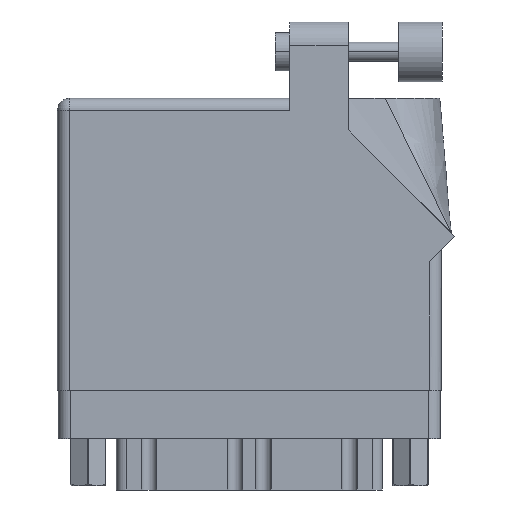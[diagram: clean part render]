
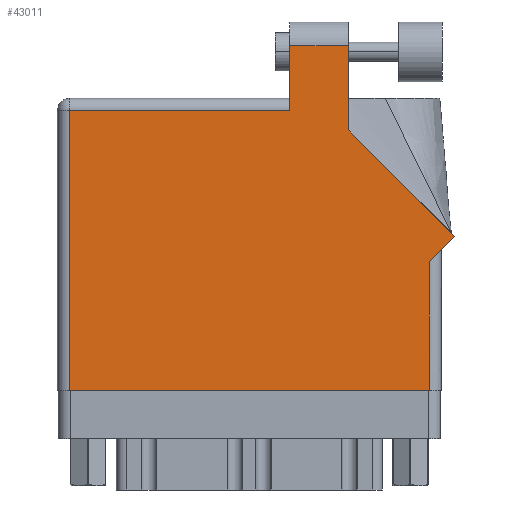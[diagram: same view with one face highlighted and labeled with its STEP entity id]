
A CAD part, front view. The second image highlights one B-rep face of the part: STEP entity #43011.
In plain terms, the highlighted face is planar.
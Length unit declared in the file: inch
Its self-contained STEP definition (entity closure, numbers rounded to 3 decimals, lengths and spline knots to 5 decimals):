
#286 = LINE ( 'NONE', #14933, #8045 ) ;
#1518 = VERTEX_POINT ( 'NONE', #29325 ) ;
#2698 = LINE ( 'NONE', #29049, #46288 ) ;
#2774 = CARTESIAN_POINT ( 'NONE',  ( 1.948, 0.737, 0. ) ) ;
#3242 = VERTEX_POINT ( 'NONE', #34035 ) ;
#4412 = LINE ( 'NONE', #15689, #27110 ) ;
#5525 = CARTESIAN_POINT ( 'NONE',  ( 1.524, 1.36442, 0. ) ) ;
#5708 = CARTESIAN_POINT ( 'NONE',  ( 1.948, 0.675, 0. ) ) ;
#6095 = EDGE_CURVE ( 'NONE', #1518, #3242, #2698, .T. ) ;
#6909 = DIRECTION ( 'NONE',  ( -1., 0., 0. ) ) ;
#7051 = CARTESIAN_POINT ( 'NONE',  ( 2.08071, 0.80771, 0. ) ) ;
#7114 = CARTESIAN_POINT ( 'NONE',  ( 0.062, 0., 0. ) ) ;
#7237 = DIRECTION ( 'NONE',  ( 0., -1., 0. ) ) ;
#7790 = EDGE_CURVE ( 'NONE', #12646, #35884, #40421, .T. ) ;
#7879 = EDGE_CURVE ( 'NONE', #41686, #40279, #4412, .T. ) ;
#8045 = VECTOR ( 'NONE', #7237, 39.37008 ) ;
#8227 = DIRECTION ( 'NONE',  ( -1., 0., 0. ) ) ;
#8655 = EDGE_CURVE ( 'NONE', #35884, #24868, #16354, .T. ) ;
#9692 = CARTESIAN_POINT ( 'NONE',  ( 0., 1.53, 0. ) ) ;
#9715 = ORIENTED_EDGE ( 'NONE', *, *, #6095, .T. ) ;
#9920 = ORIENTED_EDGE ( 'NONE', *, *, #22254, .T. ) ;
#10200 = LINE ( 'NONE', #2774, #47180 ) ;
#11770 = VECTOR ( 'NONE', #32946, 39.37008 ) ;
#12646 = VERTEX_POINT ( 'NONE', #17218 ) ;
#13825 = ORIENTED_EDGE ( 'NONE', *, *, #7879, .T. ) ;
#14439 = DIRECTION ( 'NONE',  ( 1., 0., 0. ) ) ;
#14933 = CARTESIAN_POINT ( 'NONE',  ( 1.217, 1.53, 0. ) ) ;
#15599 = VECTOR ( 'NONE', #21138, 39.37008 ) ;
#15689 = CARTESIAN_POINT ( 'NONE',  ( 0., 1.468, 0. ) ) ;
#16354 = LINE ( 'NONE', #5525, #38835 ) ;
#17140 = PLANE ( 'NONE',  #17271 ) ;
#17218 = CARTESIAN_POINT ( 'NONE',  ( 2.08071, 0.80771, 0. ) ) ;
#17271 = AXIS2_PLACEMENT_3D ( 'NONE', #9692, #24338, #28176 ) ;
#18634 = EDGE_LOOP ( 'NONE', ( #26351, #27932, #33736, #13825, #19053, #9715, #9920, #35717, #26073 ) ) ;
#19053 = ORIENTED_EDGE ( 'NONE', *, *, #24812, .T. ) ;
#19126 = CARTESIAN_POINT ( 'NONE',  ( 0.062, 1.468, 0. ) ) ;
#19299 = EDGE_CURVE ( 'NONE', #30271, #12646, #25188, .T. ) ;
#21138 = DIRECTION ( 'NONE',  ( 0.707, 0.707, 0. ) ) ;
#22254 = EDGE_CURVE ( 'NONE', #3242, #30271, #10200, .T. ) ;
#22454 = VECTOR ( 'NONE', #6909, 39.37008 ) ;
#24338 = DIRECTION ( 'NONE',  ( 0., 0., -1. ) ) ;
#24651 = DIRECTION ( 'NONE',  ( 0., -1., 0. ) ) ;
#24812 = EDGE_CURVE ( 'NONE', #40279, #1518, #47204, .T. ) ;
#24868 = VERTEX_POINT ( 'NONE', #40694 ) ;
#25167 = EDGE_CURVE ( 'NONE', #37514, #41686, #286, .T. ) ;
#25188 = LINE ( 'NONE', #35260, #15599 ) ;
#26073 = ORIENTED_EDGE ( 'NONE', *, *, #7790, .T. ) ;
#26351 = ORIENTED_EDGE ( 'NONE', *, *, #8655, .T. ) ;
#27110 = VECTOR ( 'NONE', #8227, 39.37008 ) ;
#27932 = ORIENTED_EDGE ( 'NONE', *, *, #37151, .T. ) ;
#27936 = FACE_OUTER_BOUND ( 'NONE', #18634, .T. ) ;
#28176 = DIRECTION ( 'NONE',  ( -1., 0., 0. ) ) ;
#29049 = CARTESIAN_POINT ( 'NONE',  ( 0., 0., 0. ) ) ;
#29325 = CARTESIAN_POINT ( 'NONE',  ( 0.062, 0., 0. ) ) ;
#30271 = VERTEX_POINT ( 'NONE', #5708 ) ;
#32598 = CARTESIAN_POINT ( 'NONE',  ( 1.217, 1.805, 0. ) ) ;
#32946 = DIRECTION ( 'NONE',  ( -0.707, 0.707, 0. ) ) ;
#33316 = CARTESIAN_POINT ( 'NONE',  ( 1.524, 1.36442, 0. ) ) ;
#33736 = ORIENTED_EDGE ( 'NONE', *, *, #25167, .T. ) ;
#34035 = CARTESIAN_POINT ( 'NONE',  ( 1.948, 0., 0. ) ) ;
#34056 = VECTOR ( 'NONE', #24651, 39.37008 ) ;
#35260 = CARTESIAN_POINT ( 'NONE',  ( 2.01, 0.737, 0. ) ) ;
#35263 = DIRECTION ( 'NONE',  ( 0., 1., 0. ) ) ;
#35717 = ORIENTED_EDGE ( 'NONE', *, *, #19299, .T. ) ;
#35862 = DIRECTION ( 'NONE',  ( 0., 1., 0. ) ) ;
#35884 = VERTEX_POINT ( 'NONE', #33316 ) ;
#36191 = LINE ( 'NONE', #32598, #22454 ) ;
#37151 = EDGE_CURVE ( 'NONE', #24868, #37514, #36191, .T. ) ;
#37514 = VERTEX_POINT ( 'NONE', #46236 ) ;
#38835 = VECTOR ( 'NONE', #35263, 39.37008 ) ;
#40279 = VERTEX_POINT ( 'NONE', #19126 ) ;
#40421 = LINE ( 'NONE', #7051, #11770 ) ;
#40694 = CARTESIAN_POINT ( 'NONE',  ( 1.524, 1.805, 0. ) ) ;
#41686 = VERTEX_POINT ( 'NONE', #42597 ) ;
#42597 = CARTESIAN_POINT ( 'NONE',  ( 1.217, 1.468, 0. ) ) ;
#43011 = ADVANCED_FACE ( 'NONE', ( #27936 ), #17140, .F. ) ;
#46236 = CARTESIAN_POINT ( 'NONE',  ( 1.217, 1.805, 0. ) ) ;
#46288 = VECTOR ( 'NONE', #14439, 39.37008 ) ;
#47180 = VECTOR ( 'NONE', #35862, 39.37008 ) ;
#47204 = LINE ( 'NONE', #7114, #34056 ) ;
